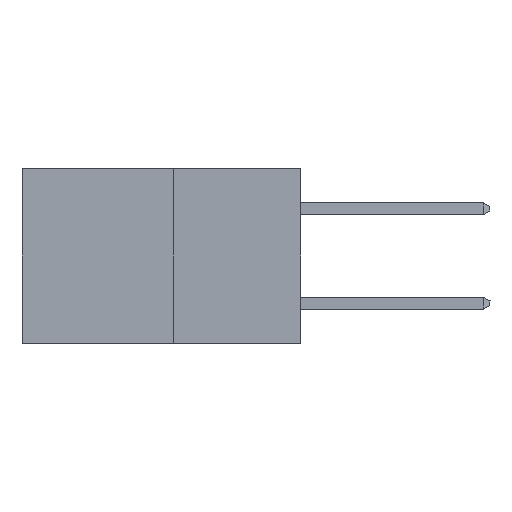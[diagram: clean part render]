
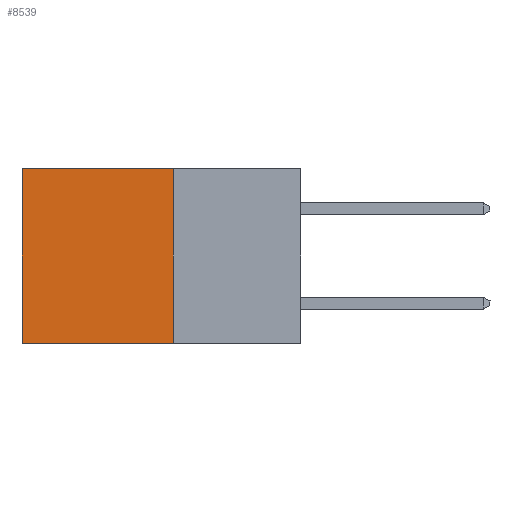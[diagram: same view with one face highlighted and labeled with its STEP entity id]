
A CAD part, left-side view. The second image highlights one B-rep face of the part: STEP entity #8539.
In plain terms, the highlighted planar face has unit normal (-1, 0, 0).
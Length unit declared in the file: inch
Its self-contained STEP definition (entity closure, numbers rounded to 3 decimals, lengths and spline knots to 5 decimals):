
#80 = CARTESIAN_POINT ( 'NONE',  ( 0.277, 0.59, 0. ) ) ;
#124 = EDGE_CURVE ( 'NONE', #6938, #145, #2742, .T. ) ;
#145 = VERTEX_POINT ( 'NONE', #80 ) ;
#232 = ORIENTED_EDGE ( 'NONE', *, *, #8133, .F. ) ;
#474 = VECTOR ( 'NONE', #3227, 39.37008 ) ;
#723 = CARTESIAN_POINT ( 'NONE',  ( 0.277, 0.27, -0.37 ) ) ;
#920 = LINE ( 'NONE', #4093, #6383 ) ;
#1329 = LINE ( 'NONE', #5429, #8445 ) ;
#1345 = VERTEX_POINT ( 'NONE', #8436 ) ;
#1661 = EDGE_CURVE ( 'NONE', #145, #7400, #1329, .T. ) ;
#2275 = DIRECTION ( 'NONE',  ( 1., 0., 0. ) ) ;
#2546 = EDGE_LOOP ( 'NONE', ( #4204, #232, #4666, #8824 ) ) ;
#2646 = LINE ( 'NONE', #4928, #6167 ) ;
#2742 = LINE ( 'NONE', #5793, #474 ) ;
#2880 = CARTESIAN_POINT ( 'NONE',  ( 0.277, 0.27, 0. ) ) ;
#2899 = EDGE_CURVE ( 'NONE', #6938, #1345, #2646, .T. ) ;
#3227 = DIRECTION ( 'NONE',  ( 0., 1., 0. ) ) ;
#3412 = AXIS2_PLACEMENT_3D ( 'NONE', #723, #2275, #7176 ) ;
#4093 = CARTESIAN_POINT ( 'NONE',  ( 0.277, 0.27, -0.37 ) ) ;
#4204 = ORIENTED_EDGE ( 'NONE', *, *, #1661, .T. ) ;
#4666 = ORIENTED_EDGE ( 'NONE', *, *, #2899, .F. ) ;
#4816 = DIRECTION ( 'NONE',  ( 0., 1., 0. ) ) ;
#4928 = CARTESIAN_POINT ( 'NONE',  ( 0.277, 0.27, -0.37 ) ) ;
#5340 = DIRECTION ( 'NONE',  ( 0., 0., -1. ) ) ;
#5429 = CARTESIAN_POINT ( 'NONE',  ( 0.277, 0.59, -0.37 ) ) ;
#5634 = DIRECTION ( 'NONE',  ( 0., 0., -1. ) ) ;
#5767 = CARTESIAN_POINT ( 'NONE',  ( 0.277, 0.59, -0.37 ) ) ;
#5793 = CARTESIAN_POINT ( 'NONE',  ( 0.277, 0.27, 0. ) ) ;
#6167 = VECTOR ( 'NONE', #5634, 39.37008 ) ;
#6383 = VECTOR ( 'NONE', #4816, 39.37008 ) ;
#6472 = PLANE ( 'NONE',  #3412 ) ;
#6938 = VERTEX_POINT ( 'NONE', #2880 ) ;
#7176 = DIRECTION ( 'NONE',  ( 0., 0., -1. ) ) ;
#7400 = VERTEX_POINT ( 'NONE', #5767 ) ;
#8046 = FACE_OUTER_BOUND ( 'NONE', #2546, .T. ) ;
#8133 = EDGE_CURVE ( 'NONE', #1345, #7400, #920, .T. ) ;
#8436 = CARTESIAN_POINT ( 'NONE',  ( 0.277, 0.27, -0.37 ) ) ;
#8445 = VECTOR ( 'NONE', #5340, 39.37008 ) ;
#8539 = ADVANCED_FACE ( 'NONE', ( #8046 ), #6472, .F. ) ;
#8824 = ORIENTED_EDGE ( 'NONE', *, *, #124, .T. ) ;
